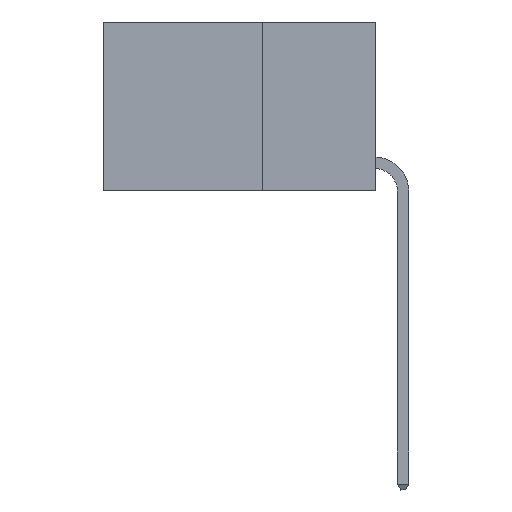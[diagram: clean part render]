
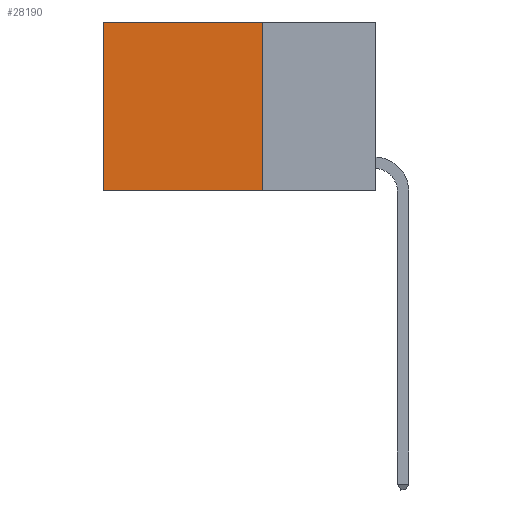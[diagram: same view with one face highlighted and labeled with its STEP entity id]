
A CAD part, left-side view. The second image highlights one B-rep face of the part: STEP entity #28190.
In plain terms, the highlighted planar face has unit normal (-1, 0, 0).
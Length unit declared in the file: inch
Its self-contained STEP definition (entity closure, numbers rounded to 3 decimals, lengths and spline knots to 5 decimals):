
#305 = ORIENTED_EDGE ( 'NONE', *, *, #2525, .T. ) ;
#1092 = VERTEX_POINT ( 'NONE', #23356 ) ;
#2525 = EDGE_CURVE ( 'NONE', #3377, #22936, #23025, .T. ) ;
#3377 = VERTEX_POINT ( 'NONE', #5553 ) ;
#5337 = EDGE_LOOP ( 'NONE', ( #305, #7432, #9936, #28064 ) ) ;
#5448 = CARTESIAN_POINT ( 'NONE',  ( 0.2625, 0.25, 0. ) ) ;
#5553 = CARTESIAN_POINT ( 'NONE',  ( 0.2625, 0.6, 0. ) ) ;
#6669 = EDGE_CURVE ( 'NONE', #9420, #1092, #25195, .T. ) ;
#7432 = ORIENTED_EDGE ( 'NONE', *, *, #20130, .F. ) ;
#8491 = LINE ( 'NONE', #17977, #28325 ) ;
#8566 = CARTESIAN_POINT ( 'NONE',  ( 0.2625, 0.25, -0.37 ) ) ;
#9420 = VERTEX_POINT ( 'NONE', #29076 ) ;
#9782 = DIRECTION ( 'NONE',  ( 0., 0., -1. ) ) ;
#9936 = ORIENTED_EDGE ( 'NONE', *, *, #6669, .F. ) ;
#10342 = VECTOR ( 'NONE', #18051, 39.37008 ) ;
#13373 = CARTESIAN_POINT ( 'NONE',  ( 0.2625, 0.25, 0. ) ) ;
#15871 = DIRECTION ( 'NONE',  ( 0., 0., -1. ) ) ;
#16176 = CARTESIAN_POINT ( 'NONE',  ( 0.2625, 0.6, 0. ) ) ;
#16956 = PLANE ( 'NONE',  #30409 ) ;
#17977 = CARTESIAN_POINT ( 'NONE',  ( 0.2625, 0.25, 0. ) ) ;
#18051 = DIRECTION ( 'NONE',  ( 0., 1., 0. ) ) ;
#20130 = EDGE_CURVE ( 'NONE', #1092, #22936, #22729, .T. ) ;
#20616 = DIRECTION ( 'NONE',  ( 0., 1., 0. ) ) ;
#22729 = LINE ( 'NONE', #8566, #10342 ) ;
#22936 = VERTEX_POINT ( 'NONE', #27002 ) ;
#23025 = LINE ( 'NONE', #16176, #24557 ) ;
#23356 = CARTESIAN_POINT ( 'NONE',  ( 0.2625, 0.25, -0.37 ) ) ;
#24106 = FACE_OUTER_BOUND ( 'NONE', #5337, .T. ) ;
#24557 = VECTOR ( 'NONE', #25655, 39.37008 ) ;
#25195 = LINE ( 'NONE', #13373, #27827 ) ;
#25655 = DIRECTION ( 'NONE',  ( 0., 0., -1. ) ) ;
#25817 = EDGE_CURVE ( 'NONE', #9420, #3377, #8491, .T. ) ;
#26131 = DIRECTION ( 'NONE',  ( 1., 0., 0. ) ) ;
#27002 = CARTESIAN_POINT ( 'NONE',  ( 0.2625, 0.6, -0.37 ) ) ;
#27827 = VECTOR ( 'NONE', #15871, 39.37008 ) ;
#28064 = ORIENTED_EDGE ( 'NONE', *, *, #25817, .T. ) ;
#28190 = ADVANCED_FACE ( 'NONE', ( #24106 ), #16956, .F. ) ;
#28325 = VECTOR ( 'NONE', #20616, 39.37008 ) ;
#29076 = CARTESIAN_POINT ( 'NONE',  ( 0.2625, 0.25, 0. ) ) ;
#30409 = AXIS2_PLACEMENT_3D ( 'NONE', #5448, #26131, #9782 ) ;
